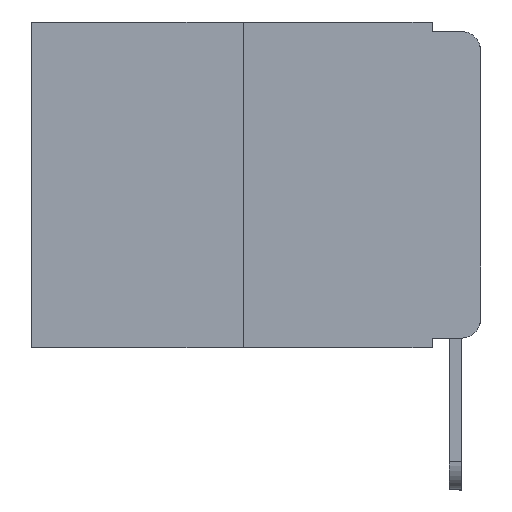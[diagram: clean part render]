
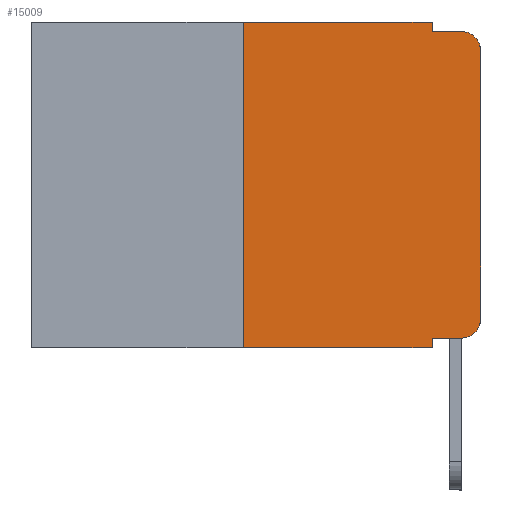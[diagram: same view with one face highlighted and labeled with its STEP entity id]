
A CAD part, left-side view. The second image highlights one B-rep face of the part: STEP entity #15009.
In plain terms, the highlighted planar face has unit normal (-1, 0, 0).
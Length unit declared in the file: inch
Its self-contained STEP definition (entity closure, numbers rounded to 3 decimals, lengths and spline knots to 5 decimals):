
#168 = CARTESIAN_POINT ( 'NONE',  ( 0., 0., -0.313 ) ) ;
#734 = VERTEX_POINT ( 'NONE', #168 ) ;
#1078 = VECTOR ( 'NONE', #12729, 39.37008 ) ;
#1223 = CARTESIAN_POINT ( 'NONE',  ( 0., 0.051, -0.333 ) ) ;
#1563 = FACE_OUTER_BOUND ( 'NONE', #22067, .T. ) ;
#2510 = EDGE_CURVE ( 'NONE', #20337, #14626, #14354, .T. ) ;
#2746 = DIRECTION ( 'NONE',  ( 0., 0., -1. ) ) ;
#3006 = LINE ( 'NONE', #11142, #24856 ) ;
#3912 = EDGE_CURVE ( 'NONE', #734, #8579, #6619, .T. ) ;
#5002 = ORIENTED_EDGE ( 'NONE', *, *, #10544, .F. ) ;
#5315 = EDGE_CURVE ( 'NONE', #16672, #20333, #21325, .T. ) ;
#6098 = CIRCLE ( 'NONE', #18696, 0.02 ) ;
#6251 = VERTEX_POINT ( 'NONE', #16806 ) ;
#6619 = LINE ( 'NONE', #14652, #7755 ) ;
#6683 = CARTESIAN_POINT ( 'NONE',  ( 0., 0.25, 0. ) ) ;
#6910 = VECTOR ( 'NONE', #16504, 39.37008 ) ;
#6920 = CARTESIAN_POINT ( 'NONE',  ( 0., 0.051, -0.01 ) ) ;
#6968 = ORIENTED_EDGE ( 'NONE', *, *, #3912, .T. ) ;
#7405 = ORIENTED_EDGE ( 'NONE', *, *, #11467, .F. ) ;
#7502 = VECTOR ( 'NONE', #22355, 39.37008 ) ;
#7755 = VECTOR ( 'NONE', #8601, 39.37008 ) ;
#7788 = CARTESIAN_POINT ( 'NONE',  ( 0., 0.02, -0.313 ) ) ;
#7920 = DIRECTION ( 'NONE',  ( -1., 0., 0. ) ) ;
#8034 = CARTESIAN_POINT ( 'NONE',  ( 0., 0.051, -0.01 ) ) ;
#8475 = DIRECTION ( 'NONE',  ( 0., 0., -1. ) ) ;
#8579 = VERTEX_POINT ( 'NONE', #12255 ) ;
#8601 = DIRECTION ( 'NONE',  ( 0., 0., 1. ) ) ;
#8881 = LINE ( 'NONE', #10578, #6910 ) ;
#9045 = LINE ( 'NONE', #6683, #1078 ) ;
#9233 = DIRECTION ( 'NONE',  ( 0., -1., 0. ) ) ;
#9738 = DIRECTION ( 'NONE',  ( 0., -1., 0. ) ) ;
#9874 = LINE ( 'NONE', #25907, #13752 ) ;
#10012 = DIRECTION ( 'NONE',  ( 0., 0., -1. ) ) ;
#10544 = EDGE_CURVE ( 'NONE', #14481, #6251, #8881, .T. ) ;
#10578 = CARTESIAN_POINT ( 'NONE',  ( 0., 0.473, 0. ) ) ;
#10762 = ORIENTED_EDGE ( 'NONE', *, *, #18532, .F. ) ;
#11142 = CARTESIAN_POINT ( 'NONE',  ( 0., 0.051, 0. ) ) ;
#11467 = EDGE_CURVE ( 'NONE', #14273, #14481, #9045, .T. ) ;
#11469 = EDGE_CURVE ( 'NONE', #8579, #14626, #6098, .T. ) ;
#11992 = CARTESIAN_POINT ( 'NONE',  ( 0., 0.25, -0.343 ) ) ;
#12050 = ORIENTED_EDGE ( 'NONE', *, *, #25794, .F. ) ;
#12058 = AXIS2_PLACEMENT_3D ( 'NONE', #16627, #14148, #8475 ) ;
#12255 = CARTESIAN_POINT ( 'NONE',  ( 0., 0., -0.03 ) ) ;
#12729 = DIRECTION ( 'NONE',  ( 0., 0., 1. ) ) ;
#13234 = ORIENTED_EDGE ( 'NONE', *, *, #19171, .T. ) ;
#13305 = CARTESIAN_POINT ( 'NONE',  ( 0., 0.25, 0. ) ) ;
#13414 = EDGE_CURVE ( 'NONE', #14273, #14174, #9874, .T. ) ;
#13752 = VECTOR ( 'NONE', #9738, 39.37008 ) ;
#13836 = DIRECTION ( 'NONE',  ( 0., 0., -1. ) ) ;
#14148 = DIRECTION ( 'NONE',  ( 1., 0., 0. ) ) ;
#14174 = VERTEX_POINT ( 'NONE', #16590 ) ;
#14260 = AXIS2_PLACEMENT_3D ( 'NONE', #7788, #7920, #10012 ) ;
#14273 = VERTEX_POINT ( 'NONE', #11992 ) ;
#14354 = LINE ( 'NONE', #8034, #7502 ) ;
#14481 = VERTEX_POINT ( 'NONE', #13305 ) ;
#14626 = VERTEX_POINT ( 'NONE', #24324 ) ;
#14652 = CARTESIAN_POINT ( 'NONE',  ( 0., 0., 0. ) ) ;
#14697 = CARTESIAN_POINT ( 'NONE',  ( 0., 0.02, -0.333 ) ) ;
#15009 = ADVANCED_FACE ( 'NONE', ( #1563 ), #17592, .F. ) ;
#16499 = ORIENTED_EDGE ( 'NONE', *, *, #13414, .T. ) ;
#16504 = DIRECTION ( 'NONE',  ( 0., -1., 0. ) ) ;
#16590 = CARTESIAN_POINT ( 'NONE',  ( 0., 0.051, -0.343 ) ) ;
#16627 = CARTESIAN_POINT ( 'NONE',  ( 0., 0.473, 0. ) ) ;
#16672 = VERTEX_POINT ( 'NONE', #25197 ) ;
#16806 = CARTESIAN_POINT ( 'NONE',  ( 0., 0.051, 0. ) ) ;
#17048 = CARTESIAN_POINT ( 'NONE',  ( 0., 0.02, -0.03 ) ) ;
#17059 = DIRECTION ( 'NONE',  ( 0., 0., -1. ) ) ;
#17592 = PLANE ( 'NONE',  #12058 ) ;
#18021 = CIRCLE ( 'NONE', #14260, 0.02 ) ;
#18532 = EDGE_CURVE ( 'NONE', #6251, #20337, #3006, .T. ) ;
#18696 = AXIS2_PLACEMENT_3D ( 'NONE', #17048, #20747, #2746 ) ;
#19171 = EDGE_CURVE ( 'NONE', #20333, #734, #18021, .T. ) ;
#19589 = LINE ( 'NONE', #25797, #20339 ) ;
#20170 = ORIENTED_EDGE ( 'NONE', *, *, #2510, .F. ) ;
#20333 = VERTEX_POINT ( 'NONE', #14697 ) ;
#20337 = VERTEX_POINT ( 'NONE', #6920 ) ;
#20339 = VECTOR ( 'NONE', #13836, 39.37008 ) ;
#20747 = DIRECTION ( 'NONE',  ( -1., 0., 0. ) ) ;
#21325 = LINE ( 'NONE', #1223, #24391 ) ;
#22067 = EDGE_LOOP ( 'NONE', ( #6968, #25798, #20170, #10762, #5002, #7405, #16499, #12050, #25465, #13234 ) ) ;
#22355 = DIRECTION ( 'NONE',  ( 0., -1., 0. ) ) ;
#24324 = CARTESIAN_POINT ( 'NONE',  ( 0., 0.02, -0.01 ) ) ;
#24391 = VECTOR ( 'NONE', #9233, 39.37008 ) ;
#24856 = VECTOR ( 'NONE', #17059, 39.37008 ) ;
#25197 = CARTESIAN_POINT ( 'NONE',  ( 0., 0.051, -0.333 ) ) ;
#25465 = ORIENTED_EDGE ( 'NONE', *, *, #5315, .T. ) ;
#25794 = EDGE_CURVE ( 'NONE', #16672, #14174, #19589, .T. ) ;
#25797 = CARTESIAN_POINT ( 'NONE',  ( 0., 0.051, 0. ) ) ;
#25798 = ORIENTED_EDGE ( 'NONE', *, *, #11469, .T. ) ;
#25907 = CARTESIAN_POINT ( 'NONE',  ( 0., 0.473, -0.343 ) ) ;
